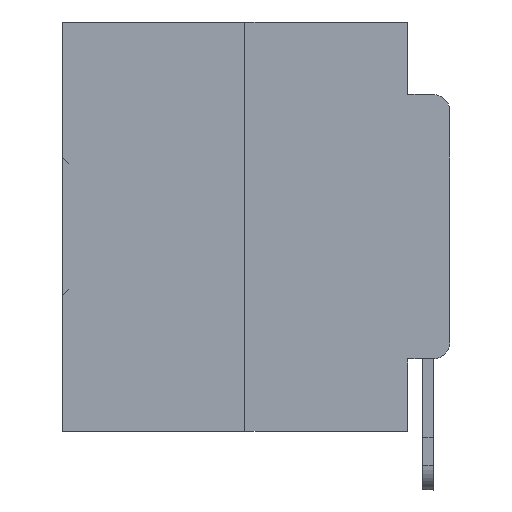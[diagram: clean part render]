
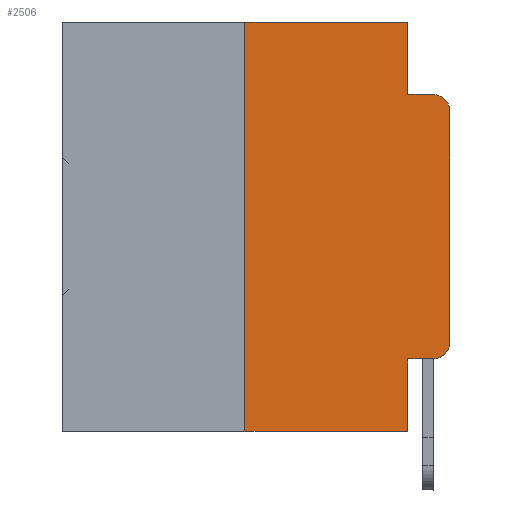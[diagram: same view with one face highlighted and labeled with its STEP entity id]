
A CAD part, left-side view. The second image highlights one B-rep face of the part: STEP entity #2506.
In plain terms, the highlighted planar face has unit normal (-1, 0, 0).
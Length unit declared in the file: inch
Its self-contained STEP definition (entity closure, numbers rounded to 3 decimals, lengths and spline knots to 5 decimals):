
#217 = VERTEX_POINT ( 'NONE', #8386 ) ;
#1188 = PLANE ( 'NONE',  #14042 ) ;
#1781 = DIRECTION ( 'NONE',  ( -1., 0., 0. ) ) ;
#2050 = VECTOR ( 'NONE', #22501, 39.37008 ) ;
#2506 = ADVANCED_FACE ( 'NONE', ( #5988 ), #1188, .F. ) ;
#2819 = EDGE_CURVE ( 'NONE', #6665, #3169, #16672, .T. ) ;
#2870 = CARTESIAN_POINT ( 'NONE',  ( 0., 0.25, -0.5 ) ) ;
#3169 = VERTEX_POINT ( 'NONE', #23758 ) ;
#3335 = VECTOR ( 'NONE', #3517, 39.37008 ) ;
#3517 = DIRECTION ( 'NONE',  ( 0., 0., -1. ) ) ;
#4366 = CARTESIAN_POINT ( 'NONE',  ( 0., 0.051, -0.0885 ) ) ;
#4632 = EDGE_CURVE ( 'NONE', #5337, #4936, #33531, .T. ) ;
#4774 = DIRECTION ( 'NONE',  ( 0., 0., -1. ) ) ;
#4936 = VERTEX_POINT ( 'NONE', #13930 ) ;
#5069 = VECTOR ( 'NONE', #16592, 39.37008 ) ;
#5337 = VERTEX_POINT ( 'NONE', #10501 ) ;
#5580 = CIRCLE ( 'NONE', #18096, 0.02 ) ;
#5654 = LINE ( 'NONE', #11519, #3335 ) ;
#5988 = FACE_OUTER_BOUND ( 'NONE', #17177, .T. ) ;
#6004 = ORIENTED_EDGE ( 'NONE', *, *, #7194, .F. ) ;
#6514 = LINE ( 'NONE', #4366, #19818 ) ;
#6665 = VERTEX_POINT ( 'NONE', #2870 ) ;
#6860 = ORIENTED_EDGE ( 'NONE', *, *, #7235, .T. ) ;
#7194 = EDGE_CURVE ( 'NONE', #6665, #28894, #11748, .T. ) ;
#7235 = EDGE_CURVE ( 'NONE', #24471, #8275, #34313, .T. ) ;
#8275 = VERTEX_POINT ( 'NONE', #18882 ) ;
#8386 = CARTESIAN_POINT ( 'NONE',  ( 0., 0.02, -0.0885 ) ) ;
#8515 = EDGE_CURVE ( 'NONE', #34704, #24471, #25622, .T. ) ;
#9087 = DIRECTION ( 'NONE',  ( 0., 0., 1. ) ) ;
#9876 = CARTESIAN_POINT ( 'NONE',  ( 0., 0., -0.1085 ) ) ;
#10041 = ORIENTED_EDGE ( 'NONE', *, *, #34901, .F. ) ;
#10501 = CARTESIAN_POINT ( 'NONE',  ( 0., 0.051, 0. ) ) ;
#10728 = VERTEX_POINT ( 'NONE', #9876 ) ;
#10904 = CARTESIAN_POINT ( 'NONE',  ( 0., 0., 0. ) ) ;
#11511 = CARTESIAN_POINT ( 'NONE',  ( 0., 0.473, -0.5 ) ) ;
#11519 = CARTESIAN_POINT ( 'NONE',  ( 0., 0.051, 0. ) ) ;
#11576 = VECTOR ( 'NONE', #9087, 39.37008 ) ;
#11686 = CARTESIAN_POINT ( 'NONE',  ( 0., 0.473, 0. ) ) ;
#11748 = LINE ( 'NONE', #17439, #11576 ) ;
#12043 = DIRECTION ( 'NONE',  ( 1., 0., 0. ) ) ;
#12098 = DIRECTION ( 'NONE',  ( -1., 0., 0. ) ) ;
#12113 = CARTESIAN_POINT ( 'NONE',  ( 0., 0.051, -0.4115 ) ) ;
#12544 = ORIENTED_EDGE ( 'NONE', *, *, #25557, .T. ) ;
#13075 = ORIENTED_EDGE ( 'NONE', *, *, #2819, .T. ) ;
#13930 = CARTESIAN_POINT ( 'NONE',  ( 0., 0.051, -0.0885 ) ) ;
#14042 = AXIS2_PLACEMENT_3D ( 'NONE', #11686, #12043, #16840 ) ;
#15226 = DIRECTION ( 'NONE',  ( 0., -1., 0. ) ) ;
#16592 = DIRECTION ( 'NONE',  ( 0., -1., 0. ) ) ;
#16672 = LINE ( 'NONE', #11511, #22573 ) ;
#16840 = DIRECTION ( 'NONE',  ( 0., 0., -1. ) ) ;
#17177 = EDGE_LOOP ( 'NONE', ( #12544, #21725, #24473, #23722, #10041, #6004, #13075, #17531, #34456, #6860 ) ) ;
#17254 = CARTESIAN_POINT ( 'NONE',  ( 0., 0.02, -0.1085 ) ) ;
#17439 = CARTESIAN_POINT ( 'NONE',  ( 0., 0.25, 0. ) ) ;
#17531 = ORIENTED_EDGE ( 'NONE', *, *, #34567, .F. ) ;
#18096 = AXIS2_PLACEMENT_3D ( 'NONE', #17254, #12098, #20451 ) ;
#18882 = CARTESIAN_POINT ( 'NONE',  ( 0., 0., -0.3915 ) ) ;
#19818 = VECTOR ( 'NONE', #15226, 39.37008 ) ;
#20009 = CARTESIAN_POINT ( 'NONE',  ( 0., 0.051, 0. ) ) ;
#20451 = DIRECTION ( 'NONE',  ( 0., 0., -1. ) ) ;
#20667 = AXIS2_PLACEMENT_3D ( 'NONE', #23642, #1781, #4774 ) ;
#21725 = ORIENTED_EDGE ( 'NONE', *, *, #34188, .T. ) ;
#22501 = DIRECTION ( 'NONE',  ( 0., 0., -1. ) ) ;
#22573 = VECTOR ( 'NONE', #29669, 39.37008 ) ;
#22953 = DIRECTION ( 'NONE',  ( 0., -1., 0. ) ) ;
#23459 = CARTESIAN_POINT ( 'NONE',  ( 0., 0.02, -0.4115 ) ) ;
#23642 = CARTESIAN_POINT ( 'NONE',  ( 0., 0.02, -0.3915 ) ) ;
#23722 = ORIENTED_EDGE ( 'NONE', *, *, #4632, .F. ) ;
#23758 = CARTESIAN_POINT ( 'NONE',  ( 0., 0.051, -0.5 ) ) ;
#24471 = VERTEX_POINT ( 'NONE', #23459 ) ;
#24473 = ORIENTED_EDGE ( 'NONE', *, *, #31693, .F. ) ;
#24956 = LINE ( 'NONE', #27986, #5069 ) ;
#25557 = EDGE_CURVE ( 'NONE', #8275, #10728, #26907, .T. ) ;
#25622 = LINE ( 'NONE', #12113, #25814 ) ;
#25814 = VECTOR ( 'NONE', #22953, 39.37008 ) ;
#26224 = CARTESIAN_POINT ( 'NONE',  ( 0., 0.051, -0.4115 ) ) ;
#26907 = LINE ( 'NONE', #10904, #31570 ) ;
#27986 = CARTESIAN_POINT ( 'NONE',  ( 0., 0.473, 0. ) ) ;
#28894 = VERTEX_POINT ( 'NONE', #29561 ) ;
#29561 = CARTESIAN_POINT ( 'NONE',  ( 0., 0.25, 0. ) ) ;
#29669 = DIRECTION ( 'NONE',  ( 0., -1., 0. ) ) ;
#29937 = DIRECTION ( 'NONE',  ( 0., 0., 1. ) ) ;
#31570 = VECTOR ( 'NONE', #29937, 39.37008 ) ;
#31693 = EDGE_CURVE ( 'NONE', #4936, #217, #6514, .T. ) ;
#33531 = LINE ( 'NONE', #20009, #2050 ) ;
#34188 = EDGE_CURVE ( 'NONE', #10728, #217, #5580, .T. ) ;
#34313 = CIRCLE ( 'NONE', #20667, 0.02 ) ;
#34456 = ORIENTED_EDGE ( 'NONE', *, *, #8515, .T. ) ;
#34567 = EDGE_CURVE ( 'NONE', #34704, #3169, #5654, .T. ) ;
#34704 = VERTEX_POINT ( 'NONE', #26224 ) ;
#34901 = EDGE_CURVE ( 'NONE', #28894, #5337, #24956, .T. ) ;
